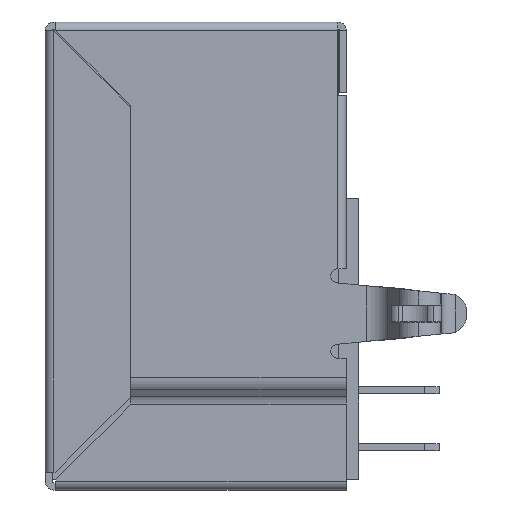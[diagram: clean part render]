
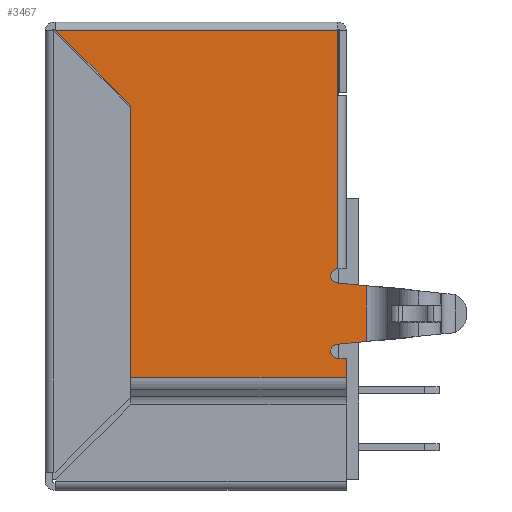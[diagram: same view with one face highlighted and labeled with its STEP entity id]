
A CAD part, left-side view. The second image highlights one B-rep face of the part: STEP entity #3467.
In plain terms, the highlighted planar face has unit normal (-1, 0, 0).
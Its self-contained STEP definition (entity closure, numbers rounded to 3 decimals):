
#395 = ORIENTED_EDGE ( 'NONE', *, *, #1681, .T. ) ;
#799 = CARTESIAN_POINT ( 'NONE',  ( -6.02, -5.31, -11.86 ) ) ;
#810 = VERTEX_POINT ( 'NONE', #2128 ) ;
#974 = LINE ( 'NONE', #15272, #7235 ) ;
#1084 = VERTEX_POINT ( 'NONE', #5645 ) ;
#1193 = ORIENTED_EDGE ( 'NONE', *, *, #6647, .F. ) ;
#1656 = DIRECTION ( 'NONE',  ( 0., 0., -1. ) ) ;
#1681 = EDGE_CURVE ( 'NONE', #810, #13735, #10583, .T. ) ;
#1821 = DIRECTION ( 'NONE',  ( 0., 0., -1. ) ) ;
#2128 = CARTESIAN_POINT ( 'NONE',  ( -6.02, -5.01, -8.7 ) ) ;
#2320 = LINE ( 'NONE', #2406, #8111 ) ;
#2406 = CARTESIAN_POINT ( 'NONE',  ( -6.02, -5.01, -11.36 ) ) ;
#2891 = VERTEX_POINT ( 'NONE', #16086 ) ;
#2978 = VERTEX_POINT ( 'NONE', #8694 ) ;
#3437 = AXIS2_PLACEMENT_3D ( 'NONE', #13129, #6583, #1656 ) ;
#3467 = ADVANCED_FACE ( 'NONE', ( #11772 ), #7886, .T. ) ;
#3648 = DIRECTION ( 'NONE',  ( 0., -1., 0. ) ) ;
#3801 = AXIS2_PLACEMENT_3D ( 'NONE', #4554, #7150, #12664 ) ;
#3907 = DIRECTION ( 'NONE',  ( 0., 0., 1. ) ) ;
#4014 = VERTEX_POINT ( 'NONE', #14269 ) ;
#4045 = VERTEX_POINT ( 'NONE', #14175 ) ;
#4047 = VECTOR ( 'NONE', #11453, 1000. ) ;
#4292 = CARTESIAN_POINT ( 'NONE',  ( -6.02, -6.012, -9.299 ) ) ;
#4465 = ORIENTED_EDGE ( 'NONE', *, *, #12336, .T. ) ;
#4554 = CARTESIAN_POINT ( 'NONE',  ( -6.02, -5.01, -8.95 ) ) ;
#4678 = VERTEX_POINT ( 'NONE', #11473 ) ;
#4795 = VECTOR ( 'NONE', #8256, 1000. ) ;
#4907 = ORIENTED_EDGE ( 'NONE', *, *, #8136, .T. ) ;
#5030 = LINE ( 'NONE', #11922, #12256 ) ;
#5093 = CARTESIAN_POINT ( 'NONE',  ( -6.02, -5.01, -11.86 ) ) ;
#5214 = LINE ( 'NONE', #9183, #15448 ) ;
#5508 = EDGE_CURVE ( 'NONE', #4045, #6918, #5030, .T. ) ;
#5536 = CARTESIAN_POINT ( 'NONE',  ( -6.02, -5.01, -0.3 ) ) ;
#5645 = CARTESIAN_POINT ( 'NONE',  ( -6.02, 2.3, -12.53 ) ) ;
#5871 = VERTEX_POINT ( 'NONE', #5093 ) ;
#6154 = CIRCLE ( 'NONE', #3437, 0.25 ) ;
#6183 = CARTESIAN_POINT ( 'NONE',  ( -6.02, -5.01, -12.775 ) ) ;
#6309 = EDGE_CURVE ( 'NONE', #13735, #7759, #10243, .T. ) ;
#6360 = DIRECTION ( 'NONE',  ( 0., -0.995, 0.098 ) ) ;
#6556 = VECTOR ( 'NONE', #3648, 1000. ) ;
#6583 = DIRECTION ( 'NONE',  ( 1., 0., 0. ) ) ;
#6598 = CARTESIAN_POINT ( 'NONE',  ( -6.02, -5.31, -12.68 ) ) ;
#6647 = EDGE_CURVE ( 'NONE', #12605, #12435, #12179, .T. ) ;
#6767 = VECTOR ( 'NONE', #1821, 1000. ) ;
#6918 = VERTEX_POINT ( 'NONE', #11218 ) ;
#7150 = DIRECTION ( 'NONE',  ( 1., 0., 0. ) ) ;
#7235 = VECTOR ( 'NONE', #11317, 1000. ) ;
#7530 = ORIENTED_EDGE ( 'NONE', *, *, #15721, .F. ) ;
#7759 = VERTEX_POINT ( 'NONE', #5536 ) ;
#7859 = ORIENTED_EDGE ( 'NONE', *, *, #6309, .T. ) ;
#7886 = PLANE ( 'NONE',  #12027 ) ;
#8111 = VECTOR ( 'NONE', #6360, 1000. ) ;
#8136 = EDGE_CURVE ( 'NONE', #6918, #4014, #10767, .T. ) ;
#8197 = EDGE_CURVE ( 'NONE', #4014, #810, #10393, .T. ) ;
#8256 = DIRECTION ( 'NONE',  ( 0., -1., 0. ) ) ;
#8694 = CARTESIAN_POINT ( 'NONE',  ( -6.02, 4.94, -0.3 ) ) ;
#9106 = CARTESIAN_POINT ( 'NONE',  ( -6.02, -6.231, -11.86 ) ) ;
#9183 = CARTESIAN_POINT ( 'NONE',  ( -6.02, 4.94, -0.3 ) ) ;
#9472 = ORIENTED_EDGE ( 'NONE', *, *, #11069, .T. ) ;
#9731 = DIRECTION ( 'NONE',  ( 0., 0.995, 0.098 ) ) ;
#9854 = CARTESIAN_POINT ( 'NONE',  ( -6.02, -5.01, -2.6 ) ) ;
#10226 = VECTOR ( 'NONE', #14342, 1000. ) ;
#10243 = LINE ( 'NONE', #6183, #4047 ) ;
#10379 = DIRECTION ( 'NONE',  ( -1., 0., 0. ) ) ;
#10393 = CIRCLE ( 'NONE', #3801, 0.25 ) ;
#10583 = LINE ( 'NONE', #13015, #11562 ) ;
#10667 = LINE ( 'NONE', #15915, #4795 ) ;
#10707 = ORIENTED_EDGE ( 'NONE', *, *, #13732, .T. ) ;
#10767 = LINE ( 'NONE', #4292, #11234 ) ;
#11069 = EDGE_CURVE ( 'NONE', #1084, #12435, #14083, .T. ) ;
#11218 = CARTESIAN_POINT ( 'NONE',  ( -6.02, -6.012, -9.299 ) ) ;
#11234 = VECTOR ( 'NONE', #9731, 1000. ) ;
#11317 = DIRECTION ( 'NONE',  ( 0., 0., -1. ) ) ;
#11453 = DIRECTION ( 'NONE',  ( 0., 0., 1. ) ) ;
#11473 = CARTESIAN_POINT ( 'NONE',  ( -6.02, -5.01, -11.36 ) ) ;
#11513 = LINE ( 'NONE', #9106, #10226 ) ;
#11562 = VECTOR ( 'NONE', #15926, 1000. ) ;
#11681 = DIRECTION ( 'NONE',  ( 0., -0.707, -0.707 ) ) ;
#11772 = FACE_OUTER_BOUND ( 'NONE', #15604, .T. ) ;
#11871 = ORIENTED_EDGE ( 'NONE', *, *, #8197, .T. ) ;
#11922 = CARTESIAN_POINT ( 'NONE',  ( -6.02, -6.012, -12.775 ) ) ;
#12027 = AXIS2_PLACEMENT_3D ( 'NONE', #13221, #10379, #3907 ) ;
#12140 = ORIENTED_EDGE ( 'NONE', *, *, #12289, .T. ) ;
#12179 = LINE ( 'NONE', #6598, #6767 ) ;
#12256 = VECTOR ( 'NONE', #15775, 1000. ) ;
#12289 = EDGE_CURVE ( 'NONE', #2978, #2891, #5214, .T. ) ;
#12336 = EDGE_CURVE ( 'NONE', #12605, #5871, #11513, .T. ) ;
#12435 = VERTEX_POINT ( 'NONE', #14680 ) ;
#12605 = VERTEX_POINT ( 'NONE', #799 ) ;
#12664 = DIRECTION ( 'NONE',  ( 0., 0., -1. ) ) ;
#12908 = ORIENTED_EDGE ( 'NONE', *, *, #15504, .T. ) ;
#13015 = CARTESIAN_POINT ( 'NONE',  ( -6.02, -5.01, -12.775 ) ) ;
#13129 = CARTESIAN_POINT ( 'NONE',  ( -6.02, -5.01, -11.61 ) ) ;
#13221 = CARTESIAN_POINT ( 'NONE',  ( -6.02, -6.231, -12.775 ) ) ;
#13732 = EDGE_CURVE ( 'NONE', #2891, #1084, #974, .T. ) ;
#13735 = VERTEX_POINT ( 'NONE', #9854 ) ;
#14083 = LINE ( 'NONE', #16765, #6556 ) ;
#14175 = CARTESIAN_POINT ( 'NONE',  ( -6.02, -6.012, -11.261 ) ) ;
#14269 = CARTESIAN_POINT ( 'NONE',  ( -6.02, -5.01, -9.2 ) ) ;
#14342 = DIRECTION ( 'NONE',  ( 0., 1., 0. ) ) ;
#14635 = ORIENTED_EDGE ( 'NONE', *, *, #5508, .T. ) ;
#14680 = CARTESIAN_POINT ( 'NONE',  ( -6.02, -5.31, -12.53 ) ) ;
#14682 = ORIENTED_EDGE ( 'NONE', *, *, #16493, .T. ) ;
#15272 = CARTESIAN_POINT ( 'NONE',  ( -6.02, 2.3, -12.775 ) ) ;
#15448 = VECTOR ( 'NONE', #11681, 1000. ) ;
#15504 = EDGE_CURVE ( 'NONE', #4678, #4045, #2320, .T. ) ;
#15604 = EDGE_LOOP ( 'NONE', ( #10707, #9472, #1193, #4465, #14682, #12908, #14635, #4907, #11871, #395, #7859, #7530, #12140 ) ) ;
#15721 = EDGE_CURVE ( 'NONE', #2978, #7759, #10667, .T. ) ;
#15775 = DIRECTION ( 'NONE',  ( 0., 0., 1. ) ) ;
#15915 = CARTESIAN_POINT ( 'NONE',  ( -6.02, -5.01, -0.3 ) ) ;
#15926 = DIRECTION ( 'NONE',  ( 0., 0., 1. ) ) ;
#16086 = CARTESIAN_POINT ( 'NONE',  ( -6.02, 2.3, -2.94 ) ) ;
#16493 = EDGE_CURVE ( 'NONE', #5871, #4678, #6154, .T. ) ;
#16765 = CARTESIAN_POINT ( 'NONE',  ( -6.02, -6.231, -12.53 ) ) ;
